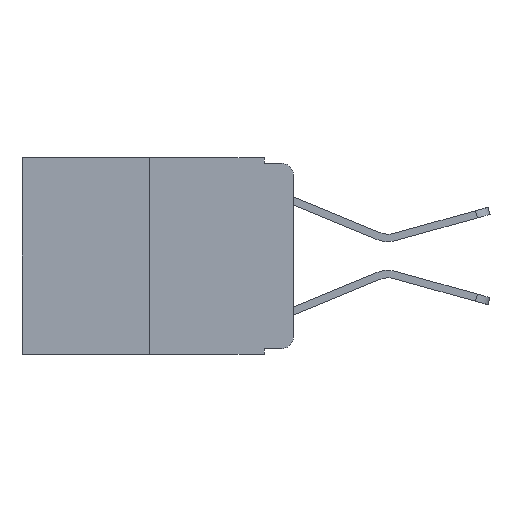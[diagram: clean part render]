
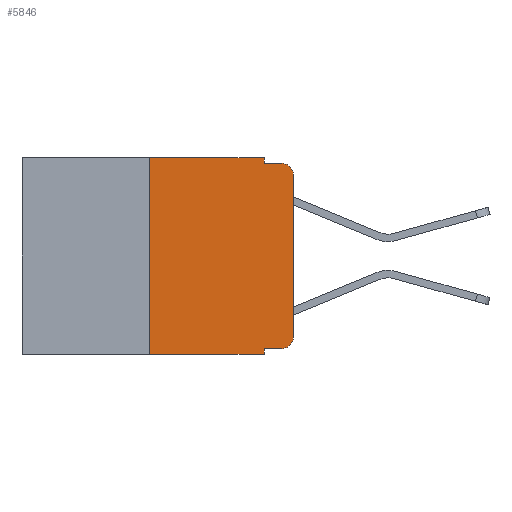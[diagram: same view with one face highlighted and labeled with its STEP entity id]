
A CAD part, left-side view. The second image highlights one B-rep face of the part: STEP entity #5846.
In plain terms, the highlighted planar face has unit normal (-1, 0, 0).
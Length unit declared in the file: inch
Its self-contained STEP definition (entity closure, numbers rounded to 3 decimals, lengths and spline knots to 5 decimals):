
#13 = VERTEX_POINT ( 'NONE', #6126 ) ;
#315 = DIRECTION ( 'NONE',  ( 0., -1., 0. ) ) ;
#371 = LINE ( 'NONE', #9830, #10176 ) ;
#470 = AXIS2_PLACEMENT_3D ( 'NONE', #8279, #2398, #5065 ) ;
#544 = AXIS2_PLACEMENT_3D ( 'NONE', #9971, #10744, #3076 ) ;
#660 = VERTEX_POINT ( 'NONE', #4812 ) ;
#830 = CARTESIAN_POINT ( 'NONE',  ( 0., 0.25, 0. ) ) ;
#884 = VERTEX_POINT ( 'NONE', #8869 ) ;
#933 = DIRECTION ( 'NONE',  ( 0., 0., -1. ) ) ;
#1163 = DIRECTION ( 'NONE',  ( 0., 0., -1. ) ) ;
#1237 = ORIENTED_EDGE ( 'NONE', *, *, #3439, .T. ) ;
#1330 = DIRECTION ( 'NONE',  ( 0., 0., -1. ) ) ;
#1442 = EDGE_CURVE ( 'NONE', #6542, #6014, #7755, .T. ) ;
#1461 = EDGE_CURVE ( 'NONE', #660, #6750, #9574, .T. ) ;
#1682 = VERTEX_POINT ( 'NONE', #8331 ) ;
#1736 = EDGE_CURVE ( 'NONE', #13, #884, #5901, .T. ) ;
#1884 = CARTESIAN_POINT ( 'NONE',  ( 0., 0.25, 0. ) ) ;
#2089 = ORIENTED_EDGE ( 'NONE', *, *, #2676, .F. ) ;
#2126 = CARTESIAN_POINT ( 'NONE',  ( 0., 0.051, 0. ) ) ;
#2398 = DIRECTION ( 'NONE',  ( -1., 0., 0. ) ) ;
#2676 = EDGE_CURVE ( 'NONE', #6750, #4589, #7090, .T. ) ;
#2962 = DIRECTION ( 'NONE',  ( 1., 0., 0. ) ) ;
#3076 = DIRECTION ( 'NONE',  ( 0., 0., -1. ) ) ;
#3173 = EDGE_LOOP ( 'NONE', ( #8651, #11003, #4215, #4374, #2089, #9874, #3534, #6832, #3902, #1237 ) ) ;
#3281 = CARTESIAN_POINT ( 'NONE',  ( 0., 0.051, -0.343 ) ) ;
#3316 = CIRCLE ( 'NONE', #470, 0.02 ) ;
#3439 = EDGE_CURVE ( 'NONE', #3761, #13, #3316, .T. ) ;
#3481 = VECTOR ( 'NONE', #4841, 39.37008 ) ;
#3507 = CARTESIAN_POINT ( 'NONE',  ( 0., 0.051, -0.01 ) ) ;
#3534 = ORIENTED_EDGE ( 'NONE', *, *, #8067, .T. ) ;
#3642 = CARTESIAN_POINT ( 'NONE',  ( 0., 0.473, 0. ) ) ;
#3761 = VERTEX_POINT ( 'NONE', #5881 ) ;
#3902 = ORIENTED_EDGE ( 'NONE', *, *, #5397, .T. ) ;
#3904 = LINE ( 'NONE', #2126, #8360 ) ;
#4215 = ORIENTED_EDGE ( 'NONE', *, *, #5428, .F. ) ;
#4286 = VECTOR ( 'NONE', #5859, 39.37008 ) ;
#4374 = ORIENTED_EDGE ( 'NONE', *, *, #4581, .F. ) ;
#4581 = EDGE_CURVE ( 'NONE', #4589, #8049, #3904, .T. ) ;
#4589 = VERTEX_POINT ( 'NONE', #7303 ) ;
#4635 = CIRCLE ( 'NONE', #544, 0.02 ) ;
#4658 = LINE ( 'NONE', #5549, #5661 ) ;
#4812 = CARTESIAN_POINT ( 'NONE',  ( 0., 0.25, -0.343 ) ) ;
#4841 = DIRECTION ( 'NONE',  ( 0., 0., 1. ) ) ;
#5065 = DIRECTION ( 'NONE',  ( 0., 0., -1. ) ) ;
#5397 = EDGE_CURVE ( 'NONE', #6542, #3761, #371, .T. ) ;
#5428 = EDGE_CURVE ( 'NONE', #8049, #1682, #4658, .T. ) ;
#5440 = VECTOR ( 'NONE', #6929, 39.37008 ) ;
#5516 = CARTESIAN_POINT ( 'NONE',  ( 0., 0.473, 0. ) ) ;
#5549 = CARTESIAN_POINT ( 'NONE',  ( 0., 0.051, -0.01 ) ) ;
#5661 = VECTOR ( 'NONE', #8029, 39.37008 ) ;
#5846 = ADVANCED_FACE ( 'NONE', ( #9026 ), #8223, .F. ) ;
#5859 = DIRECTION ( 'NONE',  ( 0., -1., 0. ) ) ;
#5881 = CARTESIAN_POINT ( 'NONE',  ( 0., 0.02, -0.333 ) ) ;
#5901 = LINE ( 'NONE', #6611, #3481 ) ;
#6014 = VERTEX_POINT ( 'NONE', #3281 ) ;
#6126 = CARTESIAN_POINT ( 'NONE',  ( 0., 0., -0.313 ) ) ;
#6542 = VERTEX_POINT ( 'NONE', #8307 ) ;
#6611 = CARTESIAN_POINT ( 'NONE',  ( 0., 0., 0. ) ) ;
#6750 = VERTEX_POINT ( 'NONE', #830 ) ;
#6832 = ORIENTED_EDGE ( 'NONE', *, *, #1442, .F. ) ;
#6929 = DIRECTION ( 'NONE',  ( 0., -1., 0. ) ) ;
#7090 = LINE ( 'NONE', #3642, #5440 ) ;
#7303 = CARTESIAN_POINT ( 'NONE',  ( 0., 0.051, 0. ) ) ;
#7592 = CARTESIAN_POINT ( 'NONE',  ( 0., 0.473, -0.343 ) ) ;
#7755 = LINE ( 'NONE', #7871, #8133 ) ;
#7871 = CARTESIAN_POINT ( 'NONE',  ( 0., 0.051, 0. ) ) ;
#7978 = EDGE_CURVE ( 'NONE', #884, #1682, #4635, .T. ) ;
#8029 = DIRECTION ( 'NONE',  ( 0., -1., 0. ) ) ;
#8049 = VERTEX_POINT ( 'NONE', #3507 ) ;
#8067 = EDGE_CURVE ( 'NONE', #660, #6014, #8407, .T. ) ;
#8133 = VECTOR ( 'NONE', #933, 39.37008 ) ;
#8223 = PLANE ( 'NONE',  #9466 ) ;
#8279 = CARTESIAN_POINT ( 'NONE',  ( 0., 0.02, -0.313 ) ) ;
#8307 = CARTESIAN_POINT ( 'NONE',  ( 0., 0.051, -0.333 ) ) ;
#8331 = CARTESIAN_POINT ( 'NONE',  ( 0., 0.02, -0.01 ) ) ;
#8360 = VECTOR ( 'NONE', #1163, 39.37008 ) ;
#8407 = LINE ( 'NONE', #7592, #4286 ) ;
#8651 = ORIENTED_EDGE ( 'NONE', *, *, #1736, .T. ) ;
#8687 = VECTOR ( 'NONE', #10464, 39.37008 ) ;
#8869 = CARTESIAN_POINT ( 'NONE',  ( 0., 0., -0.03 ) ) ;
#9026 = FACE_OUTER_BOUND ( 'NONE', #3173, .T. ) ;
#9466 = AXIS2_PLACEMENT_3D ( 'NONE', #5516, #2962, #1330 ) ;
#9574 = LINE ( 'NONE', #1884, #8687 ) ;
#9830 = CARTESIAN_POINT ( 'NONE',  ( 0., 0.051, -0.333 ) ) ;
#9874 = ORIENTED_EDGE ( 'NONE', *, *, #1461, .F. ) ;
#9971 = CARTESIAN_POINT ( 'NONE',  ( 0., 0.02, -0.03 ) ) ;
#10176 = VECTOR ( 'NONE', #315, 39.37008 ) ;
#10464 = DIRECTION ( 'NONE',  ( 0., 0., 1. ) ) ;
#10744 = DIRECTION ( 'NONE',  ( -1., 0., 0. ) ) ;
#11003 = ORIENTED_EDGE ( 'NONE', *, *, #7978, .T. ) ;
